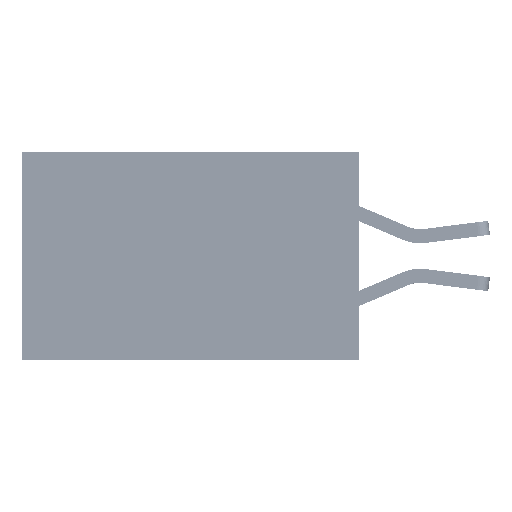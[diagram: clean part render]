
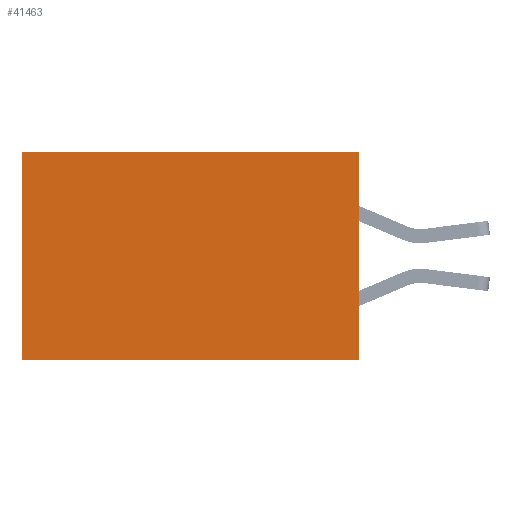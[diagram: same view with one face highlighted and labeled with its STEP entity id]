
A CAD part, left-side view. The second image highlights one B-rep face of the part: STEP entity #41463.
In plain terms, the highlighted planar face has unit normal (-1, 0, 0).
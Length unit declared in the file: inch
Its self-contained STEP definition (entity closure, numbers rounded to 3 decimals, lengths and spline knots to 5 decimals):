
#1024 = DIRECTION ( 'NONE',  ( 1., 0., 0. ) ) ;
#1767 = EDGE_LOOP ( 'NONE', ( #33122, #2587, #23651, #15841 ) ) ;
#2587 = ORIENTED_EDGE ( 'NONE', *, *, #21844, .F. ) ;
#3309 = CARTESIAN_POINT ( 'NONE',  ( 0.2875, 0., -0.37 ) ) ;
#3448 = CARTESIAN_POINT ( 'NONE',  ( 0.2875, 0.6, 0. ) ) ;
#4820 = EDGE_CURVE ( 'NONE', #41548, #41928, #31695, .T. ) ;
#7314 = VECTOR ( 'NONE', #14299, 39.37008 ) ;
#8548 = VECTOR ( 'NONE', #13964, 39.37008 ) ;
#10745 = LINE ( 'NONE', #3309, #19917 ) ;
#12980 = EDGE_CURVE ( 'NONE', #41548, #42676, #25681, .T. ) ;
#13437 = EDGE_CURVE ( 'NONE', #41928, #41905, #29111, .T. ) ;
#13964 = DIRECTION ( 'NONE',  ( 0., 0., -1. ) ) ;
#14299 = DIRECTION ( 'NONE',  ( 0., 0., -1. ) ) ;
#14927 = PLANE ( 'NONE',  #21196 ) ;
#15841 = ORIENTED_EDGE ( 'NONE', *, *, #4820, .T. ) ;
#19917 = VECTOR ( 'NONE', #20635, 39.37008 ) ;
#20635 = DIRECTION ( 'NONE',  ( 0., 1., 0. ) ) ;
#20770 = CARTESIAN_POINT ( 'NONE',  ( 0.2875, 0.6, 0. ) ) ;
#21196 = AXIS2_PLACEMENT_3D ( 'NONE', #21847, #1024, #25283 ) ;
#21844 = EDGE_CURVE ( 'NONE', #42676, #41905, #10745, .T. ) ;
#21847 = CARTESIAN_POINT ( 'NONE',  ( 0.2875, 0., 0. ) ) ;
#23651 = ORIENTED_EDGE ( 'NONE', *, *, #12980, .F. ) ;
#25283 = DIRECTION ( 'NONE',  ( 0., 0., -1. ) ) ;
#25681 = LINE ( 'NONE', #41818, #7314 ) ;
#28809 = FACE_OUTER_BOUND ( 'NONE', #1767, .T. ) ;
#29111 = LINE ( 'NONE', #3448, #8548 ) ;
#29437 = CARTESIAN_POINT ( 'NONE',  ( 0.2875, 0., 0. ) ) ;
#30592 = VECTOR ( 'NONE', #32892, 39.37008 ) ;
#31031 = CARTESIAN_POINT ( 'NONE',  ( 0.2875, 0.6, -0.37 ) ) ;
#31695 = LINE ( 'NONE', #29437, #30592 ) ;
#32892 = DIRECTION ( 'NONE',  ( 0., 1., 0. ) ) ;
#33122 = ORIENTED_EDGE ( 'NONE', *, *, #13437, .T. ) ;
#39550 = CARTESIAN_POINT ( 'NONE',  ( 0.2875, 0., 0. ) ) ;
#41463 = ADVANCED_FACE ( 'NONE', ( #28809 ), #14927, .F. ) ;
#41548 = VERTEX_POINT ( 'NONE', #39550 ) ;
#41818 = CARTESIAN_POINT ( 'NONE',  ( 0.2875, 0., 0. ) ) ;
#41905 = VERTEX_POINT ( 'NONE', #31031 ) ;
#41928 = VERTEX_POINT ( 'NONE', #20770 ) ;
#42094 = CARTESIAN_POINT ( 'NONE',  ( 0.2875, 0., -0.37 ) ) ;
#42676 = VERTEX_POINT ( 'NONE', #42094 ) ;
